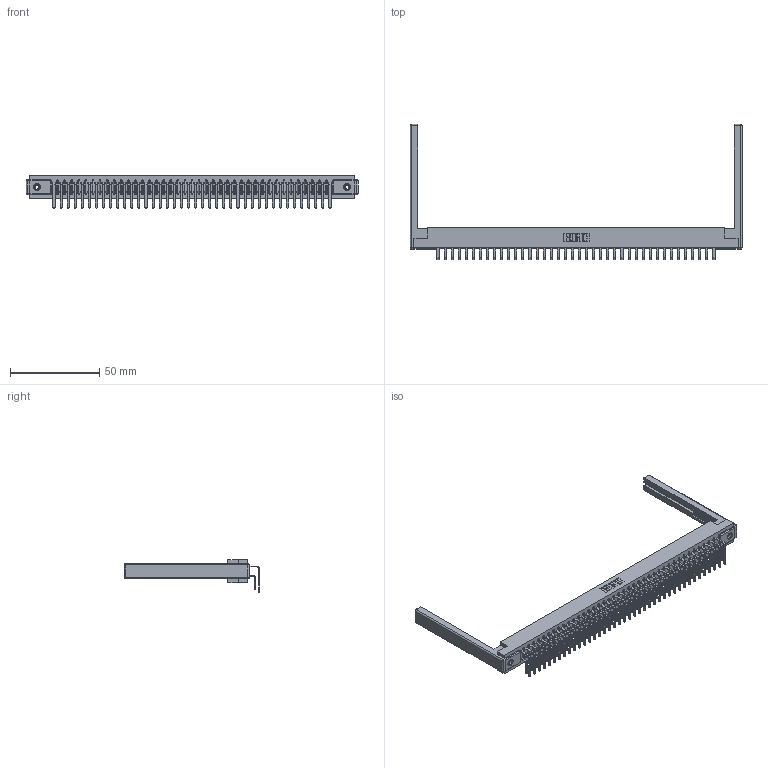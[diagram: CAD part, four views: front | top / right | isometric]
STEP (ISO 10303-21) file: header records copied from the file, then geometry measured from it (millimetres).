
FILE_DESCRIPTION (( 'STEP AP203' ), '1' );
FILE_NAME ('307-040-459-168.STEP', '2020-09-29T10:13:48', ( '' ), ( '' ), 'SwSTEP 2.0', 'SolidWorks 2020', '' );
FILE_SCHEMA (( 'CONFIG_CONTROL_DESIGN' ));
Length unit declared in the file: inch
Products named in the file (6): 307-290-001_558 559 - 1 (Single); 307-290-001_559 - 2 (Single); 307-220-068; 307-040-459-168; 345-250-001_345-250-001-102; 307 Part_.156 Dia Mounting Holes
Assembly tree (85 placements, depth 2):
  307-040-459-168
    307 Part_.156 Dia Mounting Holes
    307-290-001_558 559 - 1 (Single)  x40
    307-290-001_559 - 2 (Single)  x40
    307-220-068  x2
    345-250-001_345-250-001-102  x2
Bounding box: 185.93 x 75.65 x 18.07 mm (x, y, z)
Volume: 24492.3 mm3; surface area: 30615.6 mm2
Topology: 85 solids, 85 shells, 4313 faces, 12073 edges, 7810 vertices
Faces by surface type: plane 2798, cylinder 1409, sphere 90, cone 12, torus 4
Entity records: 40024 total; most frequent: CARTESIAN_POINT 6527, ORIENTED_EDGE 6460, DIRECTION 6408, EDGE_CURVE 3230, LINE 2474, VECTOR 2474, VERTEX_POINT 2086, AXIS2_PLACEMENT_3D 1967
